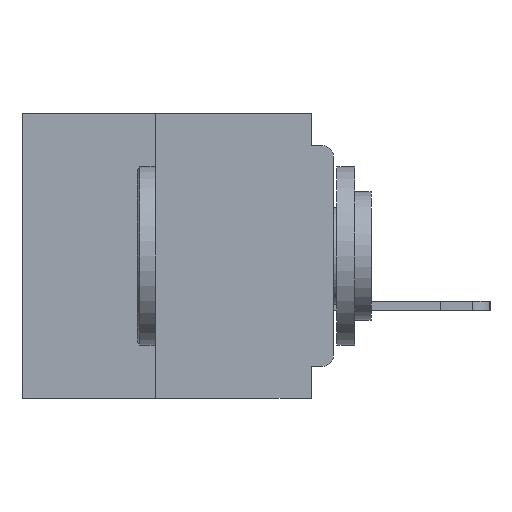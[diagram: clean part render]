
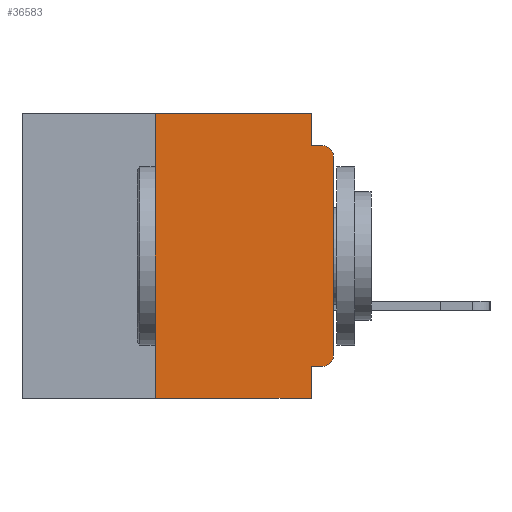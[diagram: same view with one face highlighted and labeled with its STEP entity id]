
A CAD part, left-side view. The second image highlights one B-rep face of the part: STEP entity #36583.
In plain terms, the highlighted planar face has unit normal (-1, 0, 0).
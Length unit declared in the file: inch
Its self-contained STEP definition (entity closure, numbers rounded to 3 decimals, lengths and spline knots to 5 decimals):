
#532 = EDGE_CURVE ( 'NONE', #15101, #43280, #59526, .T. ) ;
#864 = LINE ( 'NONE', #22990, #55104 ) ;
#1209 = CARTESIAN_POINT ( 'NONE',  ( 0., 0.015, -0.045 ) ) ;
#1900 = VECTOR ( 'NONE', #55029, 39.37008 ) ;
#2234 = ORIENTED_EDGE ( 'NONE', *, *, #532, .F. ) ;
#3593 = CARTESIAN_POINT ( 'NONE',  ( 0., 0.031, -0.4 ) ) ;
#3698 = CARTESIAN_POINT ( 'NONE',  ( 0., 0.437, -0.4 ) ) ;
#3881 = VECTOR ( 'NONE', #36622, 39.37008 ) ;
#4252 = CARTESIAN_POINT ( 'NONE',  ( 0., 0., -0.34 ) ) ;
#4280 = CARTESIAN_POINT ( 'NONE',  ( 0., 0.031, -0.4 ) ) ;
#4284 = CARTESIAN_POINT ( 'NONE',  ( 0., 0., -0.06 ) ) ;
#4362 = VERTEX_POINT ( 'NONE', #1209 ) ;
#5435 = VERTEX_POINT ( 'NONE', #22308 ) ;
#5503 = VERTEX_POINT ( 'NONE', #4284 ) ;
#5571 = VECTOR ( 'NONE', #8738, 39.37008 ) ;
#5633 = ORIENTED_EDGE ( 'NONE', *, *, #27548, .F. ) ;
#6851 = ORIENTED_EDGE ( 'NONE', *, *, #19506, .F. ) ;
#7169 = CARTESIAN_POINT ( 'NONE',  ( 0., 0.015, -0.06 ) ) ;
#7601 = VECTOR ( 'NONE', #54170, 39.37008 ) ;
#8738 = DIRECTION ( 'NONE',  ( 0., 0., 1. ) ) ;
#9894 = CARTESIAN_POINT ( 'NONE',  ( 0., 0.015, -0.34 ) ) ;
#11190 = CARTESIAN_POINT ( 'NONE',  ( 0., 0.437, 0. ) ) ;
#11732 = VERTEX_POINT ( 'NONE', #3593 ) ;
#11821 = DIRECTION ( 'NONE',  ( 0., 0., -1. ) ) ;
#12270 = ORIENTED_EDGE ( 'NONE', *, *, #43512, .F. ) ;
#14255 = EDGE_CURVE ( 'NONE', #5435, #29062, #43038, .T. ) ;
#14535 = DIRECTION ( 'NONE',  ( 0., 0., -1. ) ) ;
#14717 = DIRECTION ( 'NONE',  ( 0., -1., 0. ) ) ;
#15101 = VERTEX_POINT ( 'NONE', #24390 ) ;
#15315 = ORIENTED_EDGE ( 'NONE', *, *, #38569, .T. ) ;
#17166 = EDGE_CURVE ( 'NONE', #5503, #4362, #54682, .T. ) ;
#17616 = CARTESIAN_POINT ( 'NONE',  ( 0., 0.25, 0. ) ) ;
#17668 = DIRECTION ( 'NONE',  ( 0., -1., 0. ) ) ;
#18061 = CARTESIAN_POINT ( 'NONE',  ( 0., 0., -0.355 ) ) ;
#19050 = CARTESIAN_POINT ( 'NONE',  ( 0., 0.015, -0.355 ) ) ;
#19382 = CARTESIAN_POINT ( 'NONE',  ( 0., 0.437, 0. ) ) ;
#19506 = EDGE_CURVE ( 'NONE', #43280, #4362, #864, .T. ) ;
#20813 = ORIENTED_EDGE ( 'NONE', *, *, #32463, .F. ) ;
#21411 = LINE ( 'NONE', #3698, #55395 ) ;
#22308 = CARTESIAN_POINT ( 'NONE',  ( 0., 0.25, -0.4 ) ) ;
#22655 = VECTOR ( 'NONE', #57745, 39.37008 ) ;
#22990 = CARTESIAN_POINT ( 'NONE',  ( 0., 0., -0.045 ) ) ;
#23849 = FACE_OUTER_BOUND ( 'NONE', #46553, .T. ) ;
#24390 = CARTESIAN_POINT ( 'NONE',  ( 0., 0.031, 0. ) ) ;
#24915 = ORIENTED_EDGE ( 'NONE', *, *, #14255, .F. ) ;
#26496 = CARTESIAN_POINT ( 'NONE',  ( 0., 0.25, -0.4 ) ) ;
#27548 = EDGE_CURVE ( 'NONE', #55640, #11732, #39337, .T. ) ;
#27618 = DIRECTION ( 'NONE',  ( 0., -1., 0. ) ) ;
#28890 = AXIS2_PLACEMENT_3D ( 'NONE', #7169, #39521, #11821 ) ;
#29062 = VERTEX_POINT ( 'NONE', #17616 ) ;
#29822 = DIRECTION ( 'NONE',  ( 0., 0., -1. ) ) ;
#31325 = ORIENTED_EDGE ( 'NONE', *, *, #56059, .T. ) ;
#32463 = EDGE_CURVE ( 'NONE', #29062, #15101, #48747, .T. ) ;
#34847 = CARTESIAN_POINT ( 'NONE',  ( 0., 0.031, -0.045 ) ) ;
#36441 = CARTESIAN_POINT ( 'NONE',  ( 0., 0., 0. ) ) ;
#36495 = VECTOR ( 'NONE', #14717, 39.37008 ) ;
#36583 = ADVANCED_FACE ( 'NONE', ( #23849 ), #43538, .F. ) ;
#36622 = DIRECTION ( 'NONE',  ( 0., 0., -1. ) ) ;
#38569 = EDGE_CURVE ( 'NONE', #5435, #11732, #21411, .T. ) ;
#39337 = LINE ( 'NONE', #4280, #3881 ) ;
#39521 = DIRECTION ( 'NONE',  ( -1., 0., 0. ) ) ;
#40249 = LINE ( 'NONE', #18061, #1900 ) ;
#42266 = DIRECTION ( 'NONE',  ( -1., 0., 0. ) ) ;
#42854 = AXIS2_PLACEMENT_3D ( 'NONE', #9894, #42266, #14535 ) ;
#43038 = LINE ( 'NONE', #26496, #7601 ) ;
#43280 = VERTEX_POINT ( 'NONE', #34847 ) ;
#43512 = EDGE_CURVE ( 'NONE', #49130, #55640, #40249, .T. ) ;
#43538 = PLANE ( 'NONE',  #55735 ) ;
#46553 = EDGE_LOOP ( 'NONE', ( #49057, #52791, #6851, #2234, #20813, #24915, #15315, #5633, #12270, #31325 ) ) ;
#47450 = CIRCLE ( 'NONE', #42854, 0.015 ) ;
#48747 = LINE ( 'NONE', #19382, #36495 ) ;
#49057 = ORIENTED_EDGE ( 'NONE', *, *, #59558, .T. ) ;
#49130 = VERTEX_POINT ( 'NONE', #19050 ) ;
#51959 = CARTESIAN_POINT ( 'NONE',  ( 0., 0.031, -0.355 ) ) ;
#52791 = ORIENTED_EDGE ( 'NONE', *, *, #17166, .T. ) ;
#54170 = DIRECTION ( 'NONE',  ( 0., 0., 1. ) ) ;
#54682 = CIRCLE ( 'NONE', #28890, 0.015 ) ;
#54760 = LINE ( 'NONE', #36441, #5571 ) ;
#55029 = DIRECTION ( 'NONE',  ( 0., 1., 0. ) ) ;
#55104 = VECTOR ( 'NONE', #27618, 39.37008 ) ;
#55395 = VECTOR ( 'NONE', #17668, 39.37008 ) ;
#55640 = VERTEX_POINT ( 'NONE', #51959 ) ;
#55735 = AXIS2_PLACEMENT_3D ( 'NONE', #11190, #57470, #29822 ) ;
#56059 = EDGE_CURVE ( 'NONE', #49130, #57812, #47450, .T. ) ;
#57345 = CARTESIAN_POINT ( 'NONE',  ( 0., 0.031, 0. ) ) ;
#57470 = DIRECTION ( 'NONE',  ( 1., 0., 0. ) ) ;
#57745 = DIRECTION ( 'NONE',  ( 0., 0., -1. ) ) ;
#57812 = VERTEX_POINT ( 'NONE', #4252 ) ;
#59526 = LINE ( 'NONE', #57345, #22655 ) ;
#59558 = EDGE_CURVE ( 'NONE', #57812, #5503, #54760, .T. ) ;
